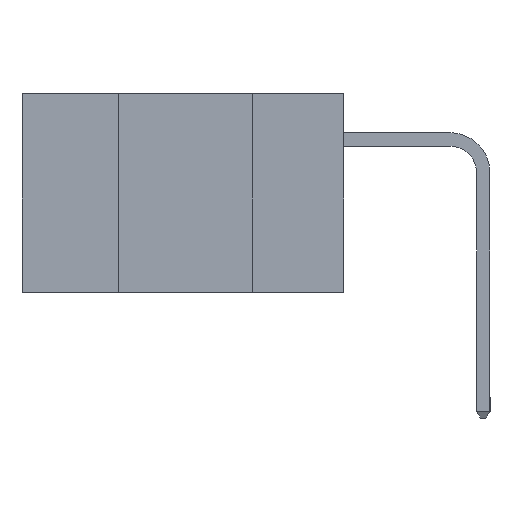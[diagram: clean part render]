
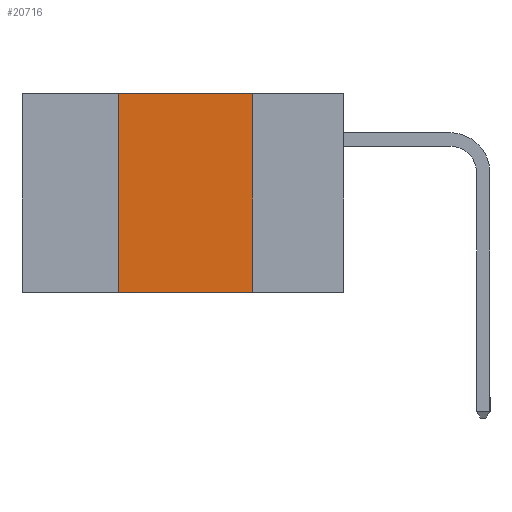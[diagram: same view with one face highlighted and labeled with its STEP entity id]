
A CAD part, left-side view. The second image highlights one B-rep face of the part: STEP entity #20716.
In plain terms, the highlighted planar face has unit normal (-1, 0, 0).
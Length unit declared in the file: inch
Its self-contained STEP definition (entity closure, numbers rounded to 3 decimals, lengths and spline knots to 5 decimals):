
#651 = VECTOR ( 'NONE', #21204, 39.37008 ) ;
#699 = EDGE_CURVE ( 'NONE', #9571, #6103, #1981, .T. ) ;
#853 = CARTESIAN_POINT ( 'NONE',  ( 0., 0.6, 0. ) ) ;
#1079 = CARTESIAN_POINT ( 'NONE',  ( 0., 0.17, 0. ) ) ;
#1981 = LINE ( 'NONE', #12580, #19679 ) ;
#2541 = EDGE_CURVE ( 'NONE', #16949, #7604, #3674, .T. ) ;
#3674 = LINE ( 'NONE', #21900, #17706 ) ;
#4442 = EDGE_CURVE ( 'NONE', #9571, #16949, #15071, .T. ) ;
#4586 = DIRECTION ( 'NONE',  ( 0., 0., -1. ) ) ;
#5125 = CARTESIAN_POINT ( 'NONE',  ( 0., 0.42, -0.37 ) ) ;
#6103 = VERTEX_POINT ( 'NONE', #14038 ) ;
#7604 = VERTEX_POINT ( 'NONE', #1079 ) ;
#9571 = VERTEX_POINT ( 'NONE', #5125 ) ;
#10218 = VECTOR ( 'NONE', #23482, 39.37008 ) ;
#11072 = LINE ( 'NONE', #15955, #651 ) ;
#11283 = ORIENTED_EDGE ( 'NONE', *, *, #699, .T. ) ;
#12197 = DIRECTION ( 'NONE',  ( 0., -1., 0. ) ) ;
#12580 = CARTESIAN_POINT ( 'NONE',  ( 0., 0.6, -0.37 ) ) ;
#13547 = AXIS2_PLACEMENT_3D ( 'NONE', #853, #15586, #4586 ) ;
#14038 = CARTESIAN_POINT ( 'NONE',  ( 0., 0.17, -0.37 ) ) ;
#15071 = LINE ( 'NONE', #23338, #10218 ) ;
#15103 = EDGE_LOOP ( 'NONE', ( #18368, #20818, #16111, #11283 ) ) ;
#15586 = DIRECTION ( 'NONE',  ( 1., 0., 0. ) ) ;
#15838 = CARTESIAN_POINT ( 'NONE',  ( 0., 0.42, 0. ) ) ;
#15955 = CARTESIAN_POINT ( 'NONE',  ( 0., 0.17, -0.37 ) ) ;
#16111 = ORIENTED_EDGE ( 'NONE', *, *, #4442, .F. ) ;
#16949 = VERTEX_POINT ( 'NONE', #15838 ) ;
#17706 = VECTOR ( 'NONE', #21854, 39.37008 ) ;
#18189 = EDGE_CURVE ( 'NONE', #7604, #6103, #11072, .T. ) ;
#18368 = ORIENTED_EDGE ( 'NONE', *, *, #18189, .F. ) ;
#19679 = VECTOR ( 'NONE', #12197, 39.37008 ) ;
#20716 = ADVANCED_FACE ( 'NONE', ( #23496 ), #20848, .F. ) ;
#20818 = ORIENTED_EDGE ( 'NONE', *, *, #2541, .F. ) ;
#20848 = PLANE ( 'NONE',  #13547 ) ;
#21204 = DIRECTION ( 'NONE',  ( 0., 0., -1. ) ) ;
#21854 = DIRECTION ( 'NONE',  ( 0., -1., 0. ) ) ;
#21900 = CARTESIAN_POINT ( 'NONE',  ( 0., 0.6, 0. ) ) ;
#23338 = CARTESIAN_POINT ( 'NONE',  ( 0., 0.42, -0.37 ) ) ;
#23482 = DIRECTION ( 'NONE',  ( 0., 0., 1. ) ) ;
#23496 = FACE_OUTER_BOUND ( 'NONE', #15103, .T. ) ;
